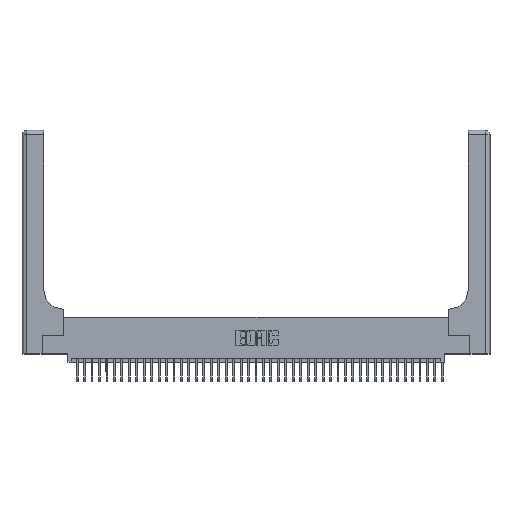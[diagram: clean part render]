
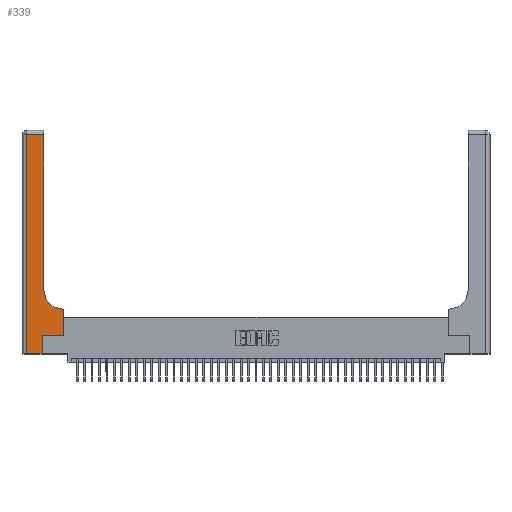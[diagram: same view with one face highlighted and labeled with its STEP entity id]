
A CAD part, top view. The second image highlights one B-rep face of the part: STEP entity #339.
In plain terms, the highlighted planar face has unit normal (0, 0, 1).
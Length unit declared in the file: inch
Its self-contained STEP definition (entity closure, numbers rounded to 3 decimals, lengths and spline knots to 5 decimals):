
#339 = ADVANCED_FACE ( 'NONE', ( #3014 ), #38844, .F. ) ;
#371 = CARTESIAN_POINT ( 'NONE',  ( 0.06, 0., 0.37 ) ) ;
#376 = LINE ( 'NONE', #34899, #33357 ) ;
#734 = DIRECTION ( 'NONE',  ( 1., 0., 0. ) ) ;
#1785 = VERTEX_POINT ( 'NONE', #24105 ) ;
#2421 = DIRECTION ( 'NONE',  ( 0., 0., -1. ) ) ;
#3002 = VECTOR ( 'NONE', #27812, 39.37008 ) ;
#3014 = FACE_OUTER_BOUND ( 'NONE', #20092, .T. ) ;
#3711 = DIRECTION ( 'NONE',  ( -1., 0., 0. ) ) ;
#3878 = EDGE_CURVE ( 'NONE', #29841, #10916, #38811, .T. ) ;
#4228 = AXIS2_PLACEMENT_3D ( 'NONE', #21687, #2421, #24940 ) ;
#4677 = VERTEX_POINT ( 'NONE', #371 ) ;
#5282 = CARTESIAN_POINT ( 'NONE',  ( 0.269, 0., 0.37 ) ) ;
#5741 = VECTOR ( 'NONE', #27744, 39.37008 ) ;
#6096 = LINE ( 'NONE', #23574, #38183 ) ;
#6156 = DIRECTION ( 'NONE',  ( 1., 0., 0. ) ) ;
#6958 = EDGE_CURVE ( 'NONE', #18987, #24337, #20195, .T. ) ;
#10249 = ORIENTED_EDGE ( 'NONE', *, *, #38019, .T. ) ;
#10552 = DIRECTION ( 'NONE',  ( 0., 1., 0. ) ) ;
#10916 = VERTEX_POINT ( 'NONE', #21651 ) ;
#12593 = VECTOR ( 'NONE', #734, 39.37008 ) ;
#12954 = ORIENTED_EDGE ( 'NONE', *, *, #3878, .T. ) ;
#12960 = ORIENTED_EDGE ( 'NONE', *, *, #30951, .T. ) ;
#14656 = LINE ( 'NONE', #38982, #12593 ) ;
#14702 = ORIENTED_EDGE ( 'NONE', *, *, #35857, .T. ) ;
#15420 = LINE ( 'NONE', #23159, #31283 ) ;
#16747 = CARTESIAN_POINT ( 'NONE',  ( 0.5585, 0.6, 0.37 ) ) ;
#16812 = EDGE_CURVE ( 'NONE', #10916, #4677, #15420, .T. ) ;
#18238 = CARTESIAN_POINT ( 'NONE',  ( 0.5585, 0.25, 0.37 ) ) ;
#18819 = DIRECTION ( 'NONE',  ( -1., 0., 0. ) ) ;
#18987 = VERTEX_POINT ( 'NONE', #27702 ) ;
#19870 = CARTESIAN_POINT ( 'NONE',  ( 0., 3., 0.37 ) ) ;
#20092 = EDGE_LOOP ( 'NONE', ( #32455, #12954, #32181, #14702, #40630, #10249, #24355, #20137, #12960 ) ) ;
#20137 = ORIENTED_EDGE ( 'NONE', *, *, #40475, .T. ) ;
#20195 = LINE ( 'NONE', #5282, #3002 ) ;
#21047 = DIRECTION ( 'NONE',  ( 0., 1., 0. ) ) ;
#21651 = CARTESIAN_POINT ( 'NONE',  ( 0.06, 2.94, 0.37 ) ) ;
#21687 = CARTESIAN_POINT ( 'NONE',  ( 0.5415, 0.85, 0.37 ) ) ;
#21816 = CARTESIAN_POINT ( 'NONE',  ( 0.2915, 0.6, 0.37 ) ) ;
#22035 = CARTESIAN_POINT ( 'NONE',  ( 0.269, 0.25, 0.37 ) ) ;
#22212 = VECTOR ( 'NONE', #18819, 39.37008 ) ;
#23053 = DIRECTION ( 'NONE',  ( 0., 0., -1. ) ) ;
#23159 = CARTESIAN_POINT ( 'NONE',  ( 0.06, 3., 0.37 ) ) ;
#23232 = LINE ( 'NONE', #21816, #22212 ) ;
#23574 = CARTESIAN_POINT ( 'NONE',  ( 0.2915, 3., 0.37 ) ) ;
#23676 = EDGE_CURVE ( 'NONE', #32202, #38182, #28730, .T. ) ;
#24105 = CARTESIAN_POINT ( 'NONE',  ( 0.2915, 0.85, 0.37 ) ) ;
#24337 = VERTEX_POINT ( 'NONE', #22035 ) ;
#24355 = ORIENTED_EDGE ( 'NONE', *, *, #23676, .T. ) ;
#24739 = CARTESIAN_POINT ( 'NONE',  ( 0.2915, 2.94, 0.37 ) ) ;
#24940 = DIRECTION ( 'NONE',  ( 1., 0., 0. ) ) ;
#27406 = CARTESIAN_POINT ( 'NONE',  ( 0.5415, 0.6, 0.37 ) ) ;
#27702 = CARTESIAN_POINT ( 'NONE',  ( 0.269, 0., 0.37 ) ) ;
#27744 = DIRECTION ( 'NONE',  ( -1., 0., 0. ) ) ;
#27812 = DIRECTION ( 'NONE',  ( 0., 1., 0. ) ) ;
#27869 = VERTEX_POINT ( 'NONE', #27406 ) ;
#28045 = AXIS2_PLACEMENT_3D ( 'NONE', #19870, #23053, #3711 ) ;
#28730 = LINE ( 'NONE', #36893, #33145 ) ;
#29841 = VERTEX_POINT ( 'NONE', #24739 ) ;
#30951 = EDGE_CURVE ( 'NONE', #27869, #1785, #38879, .T. ) ;
#31283 = VECTOR ( 'NONE', #35909, 39.37008 ) ;
#32181 = ORIENTED_EDGE ( 'NONE', *, *, #16812, .T. ) ;
#32202 = VERTEX_POINT ( 'NONE', #18238 ) ;
#32455 = ORIENTED_EDGE ( 'NONE', *, *, #39599, .T. ) ;
#33145 = VECTOR ( 'NONE', #21047, 39.37008 ) ;
#33357 = VECTOR ( 'NONE', #6156, 39.37008 ) ;
#34899 = CARTESIAN_POINT ( 'NONE',  ( 0.269, 0.25, 0.37 ) ) ;
#35857 = EDGE_CURVE ( 'NONE', #4677, #18987, #14656, .T. ) ;
#35909 = DIRECTION ( 'NONE',  ( 0., -1., 0. ) ) ;
#36893 = CARTESIAN_POINT ( 'NONE',  ( 0.5585, 0.25, 0.37 ) ) ;
#38019 = EDGE_CURVE ( 'NONE', #24337, #32202, #376, .T. ) ;
#38182 = VERTEX_POINT ( 'NONE', #16747 ) ;
#38183 = VECTOR ( 'NONE', #10552, 39.37008 ) ;
#38811 = LINE ( 'NONE', #40470, #5741 ) ;
#38844 = PLANE ( 'NONE',  #28045 ) ;
#38879 = CIRCLE ( 'NONE', #4228, 0.25 ) ;
#38982 = CARTESIAN_POINT ( 'NONE',  ( 0., 0., 0.37 ) ) ;
#39599 = EDGE_CURVE ( 'NONE', #1785, #29841, #6096, .T. ) ;
#40470 = CARTESIAN_POINT ( 'NONE',  ( 0., 2.94, 0.37 ) ) ;
#40475 = EDGE_CURVE ( 'NONE', #38182, #27869, #23232, .T. ) ;
#40630 = ORIENTED_EDGE ( 'NONE', *, *, #6958, .T. ) ;
